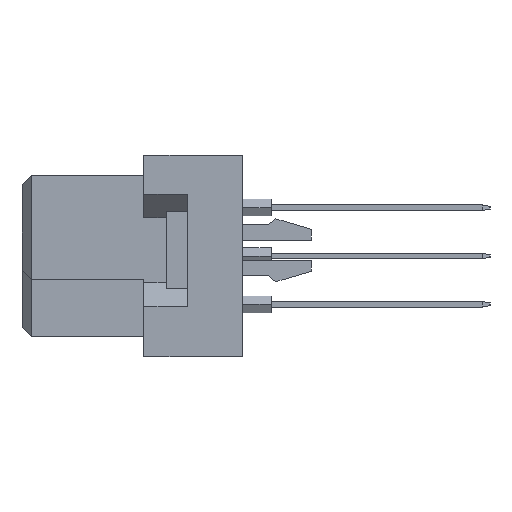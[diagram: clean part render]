
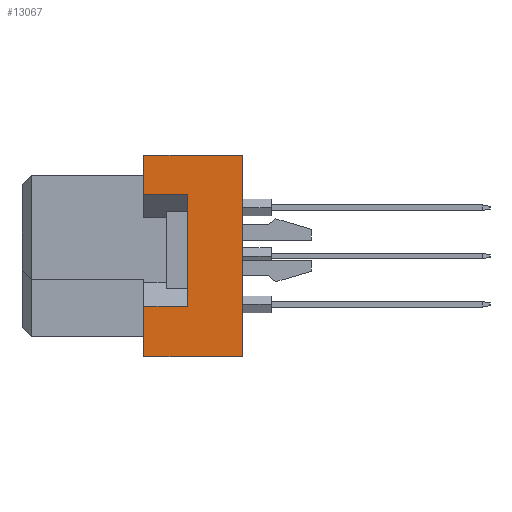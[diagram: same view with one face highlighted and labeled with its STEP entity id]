
A CAD part, left-side view. The second image highlights one B-rep face of the part: STEP entity #13067.
In plain terms, the highlighted planar face has unit normal (-1, 0, 0).
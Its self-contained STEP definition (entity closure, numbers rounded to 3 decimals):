
#64 = CARTESIAN_POINT ( 'NONE',  ( -47.5, -8.7, -2.65 ) ) ;
#1140 = EDGE_CURVE ( 'NONE', #7966, #16937, #13621, .T. ) ;
#1245 = LINE ( 'NONE', #31621, #31519 ) ;
#2691 = DIRECTION ( 'NONE',  ( 0., 0., 1. ) ) ;
#3432 = DIRECTION ( 'NONE',  ( 0., 0., 1. ) ) ;
#4578 = DIRECTION ( 'NONE',  ( 0., 1., 0. ) ) ;
#4783 = VECTOR ( 'NONE', #4578, 1000. ) ;
#5169 = EDGE_CURVE ( 'NONE', #19448, #7966, #38301, .T. ) ;
#5956 = VERTEX_POINT ( 'NONE', #14553 ) ;
#6006 = ORIENTED_EDGE ( 'NONE', *, *, #26923, .T. ) ;
#7181 = ORIENTED_EDGE ( 'NONE', *, *, #15690, .T. ) ;
#7694 = DIRECTION ( 'NONE',  ( 0., 1., 0. ) ) ;
#7807 = ORIENTED_EDGE ( 'NONE', *, *, #1140, .F. ) ;
#7966 = VERTEX_POINT ( 'NONE', #23151 ) ;
#7993 = VERTEX_POINT ( 'NONE', #13215 ) ;
#8234 = CARTESIAN_POINT ( 'NONE',  ( -47.5, -8.7, -2.65 ) ) ;
#9561 = CARTESIAN_POINT ( 'NONE',  ( -47.5, -11.6, 5.3 ) ) ;
#9567 = EDGE_LOOP ( 'NONE', ( #7181, #11977, #31046, #10734, #6006, #14835, #7807, #39821 ) ) ;
#9797 = CARTESIAN_POINT ( 'NONE',  ( -47.5, -6.4, -5.3 ) ) ;
#10203 = DIRECTION ( 'NONE',  ( -1., 0., 0. ) ) ;
#10734 = ORIENTED_EDGE ( 'NONE', *, *, #24496, .T. ) ;
#11977 = ORIENTED_EDGE ( 'NONE', *, *, #40384, .F. ) ;
#13067 = ADVANCED_FACE ( 'NONE', ( #30058 ), #39153, .T. ) ;
#13215 = CARTESIAN_POINT ( 'NONE',  ( -47.5, -11.6, -5.3 ) ) ;
#13621 = LINE ( 'NONE', #26720, #38644 ) ;
#13800 = CARTESIAN_POINT ( 'NONE',  ( -47.5, -11.6, 5.3 ) ) ;
#14496 = LINE ( 'NONE', #27164, #4783 ) ;
#14553 = CARTESIAN_POINT ( 'NONE',  ( -47.5, -11.6, 5.3 ) ) ;
#14835 = ORIENTED_EDGE ( 'NONE', *, *, #25527, .F. ) ;
#15074 = VECTOR ( 'NONE', #16556, 1000. ) ;
#15690 = EDGE_CURVE ( 'NONE', #19448, #30749, #31322, .T. ) ;
#16556 = DIRECTION ( 'NONE',  ( 0., 0., 1. ) ) ;
#16702 = CARTESIAN_POINT ( 'NONE',  ( -47.5, -6.4, -5.3 ) ) ;
#16937 = VERTEX_POINT ( 'NONE', #39210 ) ;
#17222 = CARTESIAN_POINT ( 'NONE',  ( -47.5, -6.4, -2.65 ) ) ;
#19448 = VERTEX_POINT ( 'NONE', #8234 ) ;
#20294 = VECTOR ( 'NONE', #22456, 1000. ) ;
#22255 = VECTOR ( 'NONE', #36839, 1000. ) ;
#22456 = DIRECTION ( 'NONE',  ( 0., 1., 0. ) ) ;
#22769 = AXIS2_PLACEMENT_3D ( 'NONE', #13800, #10203, #23525 ) ;
#23151 = CARTESIAN_POINT ( 'NONE',  ( -47.5, -8.7, 3.25 ) ) ;
#23525 = DIRECTION ( 'NONE',  ( 0., 0., 1. ) ) ;
#23956 = CARTESIAN_POINT ( 'NONE',  ( -47.5, -6.4, -5.3 ) ) ;
#24365 = LINE ( 'NONE', #23956, #22255 ) ;
#24496 = EDGE_CURVE ( 'NONE', #7993, #5956, #1245, .T. ) ;
#25527 = EDGE_CURVE ( 'NONE', #16937, #31412, #24365, .T. ) ;
#26465 = EDGE_CURVE ( 'NONE', #7993, #28808, #14496, .T. ) ;
#26720 = CARTESIAN_POINT ( 'NONE',  ( -47.5, -8.7, 3.25 ) ) ;
#26923 = EDGE_CURVE ( 'NONE', #5956, #31412, #31738, .T. ) ;
#27164 = CARTESIAN_POINT ( 'NONE',  ( -47.5, -11.6, -5.3 ) ) ;
#28808 = VERTEX_POINT ( 'NONE', #16702 ) ;
#29010 = LINE ( 'NONE', #9797, #15074 ) ;
#29365 = CARTESIAN_POINT ( 'NONE',  ( -47.5, -6.4, 5.3 ) ) ;
#30058 = FACE_OUTER_BOUND ( 'NONE', #9567, .T. ) ;
#30749 = VERTEX_POINT ( 'NONE', #17222 ) ;
#31046 = ORIENTED_EDGE ( 'NONE', *, *, #26465, .F. ) ;
#31322 = LINE ( 'NONE', #34280, #36567 ) ;
#31412 = VERTEX_POINT ( 'NONE', #29365 ) ;
#31519 = VECTOR ( 'NONE', #2691, 1000. ) ;
#31621 = CARTESIAN_POINT ( 'NONE',  ( -47.5, -11.6, 5.3 ) ) ;
#31738 = LINE ( 'NONE', #9561, #20294 ) ;
#34280 = CARTESIAN_POINT ( 'NONE',  ( -47.5, -8.7, -2.65 ) ) ;
#34486 = DIRECTION ( 'NONE',  ( 0., 1., 0. ) ) ;
#35437 = VECTOR ( 'NONE', #3432, 1000. ) ;
#36567 = VECTOR ( 'NONE', #34486, 1000. ) ;
#36839 = DIRECTION ( 'NONE',  ( 0., 0., 1. ) ) ;
#38301 = LINE ( 'NONE', #64, #35437 ) ;
#38644 = VECTOR ( 'NONE', #7694, 1000. ) ;
#39153 = PLANE ( 'NONE',  #22769 ) ;
#39210 = CARTESIAN_POINT ( 'NONE',  ( -47.5, -6.4, 3.25 ) ) ;
#39821 = ORIENTED_EDGE ( 'NONE', *, *, #5169, .F. ) ;
#40384 = EDGE_CURVE ( 'NONE', #28808, #30749, #29010, .T. ) ;
